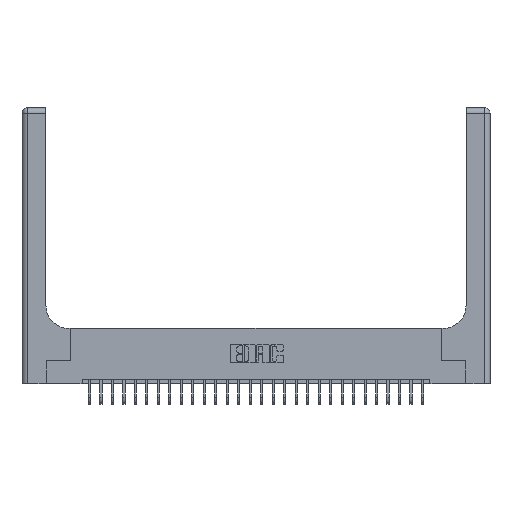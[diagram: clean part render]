
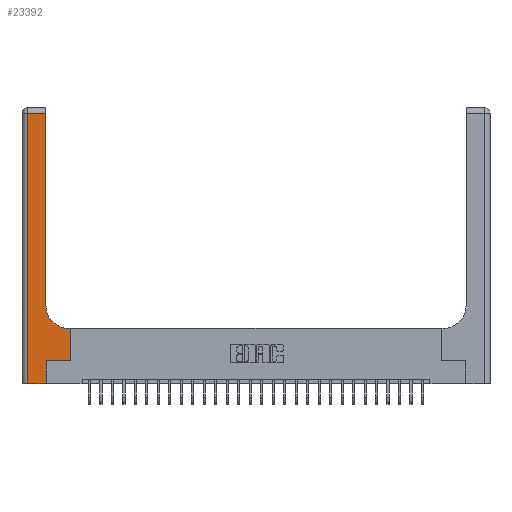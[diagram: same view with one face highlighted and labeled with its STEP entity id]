
A CAD part, top view. The second image highlights one B-rep face of the part: STEP entity #23392.
In plain terms, the highlighted planar face has unit normal (0, 0, 1).
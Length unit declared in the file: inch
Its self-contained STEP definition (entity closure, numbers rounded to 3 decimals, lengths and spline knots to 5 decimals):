
#844 = VERTEX_POINT ( 'NONE', #16510 ) ;
#870 = CARTESIAN_POINT ( 'NONE',  ( 0.265, 0., 0.37 ) ) ;
#1686 = LINE ( 'NONE', #24046, #26353 ) ;
#2075 = DIRECTION ( 'NONE',  ( 0., 0., -1. ) ) ;
#2147 = ORIENTED_EDGE ( 'NONE', *, *, #7878, .T. ) ;
#3045 = LINE ( 'NONE', #11884, #12240 ) ;
#3277 = EDGE_CURVE ( 'NONE', #5269, #13275, #16697, .T. ) ;
#3572 = DIRECTION ( 'NONE',  ( -1., 0., 0. ) ) ;
#5269 = VERTEX_POINT ( 'NONE', #870 ) ;
#5287 = ORIENTED_EDGE ( 'NONE', *, *, #12904, .T. ) ;
#5289 = VECTOR ( 'NONE', #7832, 39.37008 ) ;
#6497 = VECTOR ( 'NONE', #19755, 39.37008 ) ;
#6749 = CARTESIAN_POINT ( 'NONE',  ( 0.26, 0.85, 0.37 ) ) ;
#6886 = EDGE_CURVE ( 'NONE', #13275, #18081, #1686, .T. ) ;
#6921 = EDGE_CURVE ( 'NONE', #26466, #12293, #28215, .T. ) ;
#7120 = EDGE_CURVE ( 'NONE', #8826, #25032, #13440, .T. ) ;
#7832 = DIRECTION ( 'NONE',  ( -1., 0., 0. ) ) ;
#7845 = VECTOR ( 'NONE', #12713, 39.37008 ) ;
#7878 = EDGE_CURVE ( 'NONE', #18081, #12729, #8573, .T. ) ;
#8059 = VECTOR ( 'NONE', #3572, 39.37008 ) ;
#8478 = LINE ( 'NONE', #18949, #8059 ) ;
#8573 = LINE ( 'NONE', #17414, #6497 ) ;
#8826 = VERTEX_POINT ( 'NONE', #6749 ) ;
#11381 = CARTESIAN_POINT ( 'NONE',  ( 0.26, 3., 0.37 ) ) ;
#11884 = CARTESIAN_POINT ( 'NONE',  ( 0., 0., 0.37 ) ) ;
#11890 = VECTOR ( 'NONE', #25289, 39.37008 ) ;
#12096 = DIRECTION ( 'NONE',  ( -1., 0., 0. ) ) ;
#12240 = VECTOR ( 'NONE', #16509, 39.37008 ) ;
#12293 = VERTEX_POINT ( 'NONE', #27113 ) ;
#12580 = DIRECTION ( 'NONE',  ( 1., 0., 0. ) ) ;
#12713 = DIRECTION ( 'NONE',  ( 0., -1., 0. ) ) ;
#12729 = VERTEX_POINT ( 'NONE', #26506 ) ;
#12904 = EDGE_CURVE ( 'NONE', #12729, #844, #8478, .T. ) ;
#13009 = CARTESIAN_POINT ( 'NONE',  ( 0.06, 3., 0.37 ) ) ;
#13275 = VERTEX_POINT ( 'NONE', #23125 ) ;
#13440 = LINE ( 'NONE', #11381, #24060 ) ;
#13744 = ORIENTED_EDGE ( 'NONE', *, *, #13845, .T. ) ;
#13759 = EDGE_CURVE ( 'NONE', #12293, #5269, #3045, .T. ) ;
#13845 = EDGE_CURVE ( 'NONE', #25032, #26466, #16787, .T. ) ;
#13857 = FACE_OUTER_BOUND ( 'NONE', #26615, .T. ) ;
#14335 = CARTESIAN_POINT ( 'NONE',  ( 0.528, 0.25, 0.37 ) ) ;
#15843 = DIRECTION ( 'NONE',  ( 1., 0., 0. ) ) ;
#16509 = DIRECTION ( 'NONE',  ( 1., 0., 0. ) ) ;
#16510 = CARTESIAN_POINT ( 'NONE',  ( 0.51, 0.6, 0.37 ) ) ;
#16697 = LINE ( 'NONE', #25706, #11890 ) ;
#16787 = LINE ( 'NONE', #21156, #5289 ) ;
#17414 = CARTESIAN_POINT ( 'NONE',  ( 0.528, 0.25, 0.37 ) ) ;
#18081 = VERTEX_POINT ( 'NONE', #14335 ) ;
#18140 = ORIENTED_EDGE ( 'NONE', *, *, #3277, .T. ) ;
#18640 = CIRCLE ( 'NONE', #25583, 0.25 ) ;
#18949 = CARTESIAN_POINT ( 'NONE',  ( 0.26, 0.6, 0.37 ) ) ;
#19599 = ORIENTED_EDGE ( 'NONE', *, *, #6921, .T. ) ;
#19755 = DIRECTION ( 'NONE',  ( 0., 1., 0. ) ) ;
#20065 = CARTESIAN_POINT ( 'NONE',  ( 0.51, 0.85, 0.37 ) ) ;
#20940 = PLANE ( 'NONE',  #27876 ) ;
#21156 = CARTESIAN_POINT ( 'NONE',  ( 0., 2.94, 0.37 ) ) ;
#22294 = DIRECTION ( 'NONE',  ( 0., 1., 0. ) ) ;
#22425 = ORIENTED_EDGE ( 'NONE', *, *, #13759, .T. ) ;
#22702 = CARTESIAN_POINT ( 'NONE',  ( 0., 3., 0.37 ) ) ;
#23125 = CARTESIAN_POINT ( 'NONE',  ( 0.265, 0.25, 0.37 ) ) ;
#23392 = ADVANCED_FACE ( 'NONE', ( #13857 ), #20940, .F. ) ;
#23707 = EDGE_CURVE ( 'NONE', #844, #8826, #18640, .T. ) ;
#24046 = CARTESIAN_POINT ( 'NONE',  ( 0.265, 0.25, 0.37 ) ) ;
#24060 = VECTOR ( 'NONE', #22294, 39.37008 ) ;
#24868 = CARTESIAN_POINT ( 'NONE',  ( 0.06, 2.94, 0.37 ) ) ;
#25032 = VERTEX_POINT ( 'NONE', #28027 ) ;
#25289 = DIRECTION ( 'NONE',  ( 0., 1., 0. ) ) ;
#25457 = DIRECTION ( 'NONE',  ( 0., 0., -1. ) ) ;
#25583 = AXIS2_PLACEMENT_3D ( 'NONE', #20065, #2075, #15843 ) ;
#25706 = CARTESIAN_POINT ( 'NONE',  ( 0.265, 0., 0.37 ) ) ;
#25969 = ORIENTED_EDGE ( 'NONE', *, *, #23707, .T. ) ;
#26077 = ORIENTED_EDGE ( 'NONE', *, *, #6886, .T. ) ;
#26353 = VECTOR ( 'NONE', #12580, 39.37008 ) ;
#26466 = VERTEX_POINT ( 'NONE', #24868 ) ;
#26506 = CARTESIAN_POINT ( 'NONE',  ( 0.528, 0.6, 0.37 ) ) ;
#26615 = EDGE_LOOP ( 'NONE', ( #28090, #13744, #19599, #22425, #18140, #26077, #2147, #5287, #25969 ) ) ;
#27113 = CARTESIAN_POINT ( 'NONE',  ( 0.06, 0., 0.37 ) ) ;
#27876 = AXIS2_PLACEMENT_3D ( 'NONE', #22702, #25457, #12096 ) ;
#28027 = CARTESIAN_POINT ( 'NONE',  ( 0.26, 2.94, 0.37 ) ) ;
#28090 = ORIENTED_EDGE ( 'NONE', *, *, #7120, .T. ) ;
#28215 = LINE ( 'NONE', #13009, #7845 ) ;
